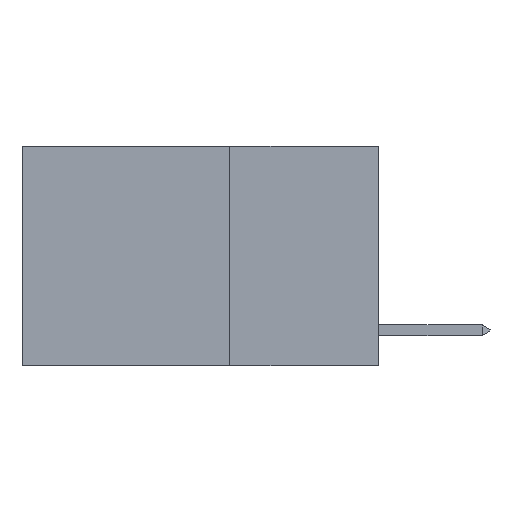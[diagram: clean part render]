
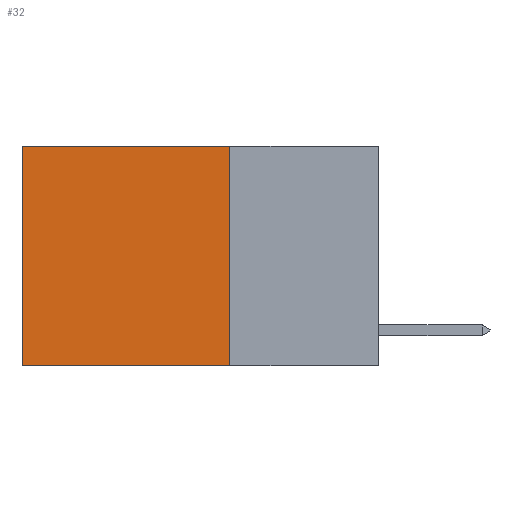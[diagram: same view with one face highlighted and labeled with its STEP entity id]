
A CAD part, left-side view. The second image highlights one B-rep face of the part: STEP entity #32.
In plain terms, the highlighted planar face has unit normal (-1, 0, 0).
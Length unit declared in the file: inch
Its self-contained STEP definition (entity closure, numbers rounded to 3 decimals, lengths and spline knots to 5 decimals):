
#32 = ADVANCED_FACE ( 'NONE', ( #9417 ), #6399, .F. ) ;
#1438 = CARTESIAN_POINT ( 'NONE',  ( 0.2625, 0.25, -0.37 ) ) ;
#1584 = CARTESIAN_POINT ( 'NONE',  ( 0.2625, 0.6, 0. ) ) ;
#1600 = VERTEX_POINT ( 'NONE', #11764 ) ;
#2020 = LINE ( 'NONE', #8127, #12349 ) ;
#2178 = ORIENTED_EDGE ( 'NONE', *, *, #5550, .F. ) ;
#2295 = CARTESIAN_POINT ( 'NONE',  ( 0.2625, 0.25, 0. ) ) ;
#2381 = EDGE_CURVE ( 'NONE', #1600, #6681, #11585, .T. ) ;
#4581 = DIRECTION ( 'NONE',  ( 1., 0., 0. ) ) ;
#4745 = EDGE_LOOP ( 'NONE', ( #11409, #2178, #5794, #10267 ) ) ;
#5550 = EDGE_CURVE ( 'NONE', #9930, #6681, #2020, .T. ) ;
#5777 = DIRECTION ( 'NONE',  ( 0., 0., -1. ) ) ;
#5794 = ORIENTED_EDGE ( 'NONE', *, *, #9414, .F. ) ;
#5984 = VECTOR ( 'NONE', #12255, 39.37008 ) ;
#6399 = PLANE ( 'NONE',  #11438 ) ;
#6413 = VECTOR ( 'NONE', #12570, 39.37008 ) ;
#6681 = VERTEX_POINT ( 'NONE', #7695 ) ;
#7588 = CARTESIAN_POINT ( 'NONE',  ( 0.2625, 0.25, 0. ) ) ;
#7695 = CARTESIAN_POINT ( 'NONE',  ( 0.2625, 0.6, -0.37 ) ) ;
#8127 = CARTESIAN_POINT ( 'NONE',  ( 0.2625, 0.25, -0.37 ) ) ;
#8243 = LINE ( 'NONE', #2295, #5984 ) ;
#9111 = VERTEX_POINT ( 'NONE', #11287 ) ;
#9414 = EDGE_CURVE ( 'NONE', #9111, #9930, #10929, .T. ) ;
#9417 = FACE_OUTER_BOUND ( 'NONE', #4745, .T. ) ;
#9550 = VECTOR ( 'NONE', #5777, 39.37008 ) ;
#9930 = VERTEX_POINT ( 'NONE', #1438 ) ;
#10267 = ORIENTED_EDGE ( 'NONE', *, *, #12968, .T. ) ;
#10929 = LINE ( 'NONE', #12973, #9550 ) ;
#11287 = CARTESIAN_POINT ( 'NONE',  ( 0.2625, 0.25, 0. ) ) ;
#11409 = ORIENTED_EDGE ( 'NONE', *, *, #2381, .T. ) ;
#11438 = AXIS2_PLACEMENT_3D ( 'NONE', #7588, #4581, #12592 ) ;
#11585 = LINE ( 'NONE', #1584, #6413 ) ;
#11764 = CARTESIAN_POINT ( 'NONE',  ( 0.2625, 0.6, 0. ) ) ;
#12255 = DIRECTION ( 'NONE',  ( 0., 1., 0. ) ) ;
#12349 = VECTOR ( 'NONE', #12941, 39.37008 ) ;
#12570 = DIRECTION ( 'NONE',  ( 0., 0., -1. ) ) ;
#12592 = DIRECTION ( 'NONE',  ( 0., 0., -1. ) ) ;
#12941 = DIRECTION ( 'NONE',  ( 0., 1., 0. ) ) ;
#12968 = EDGE_CURVE ( 'NONE', #9111, #1600, #8243, .T. ) ;
#12973 = CARTESIAN_POINT ( 'NONE',  ( 0.2625, 0.25, 0. ) ) ;
